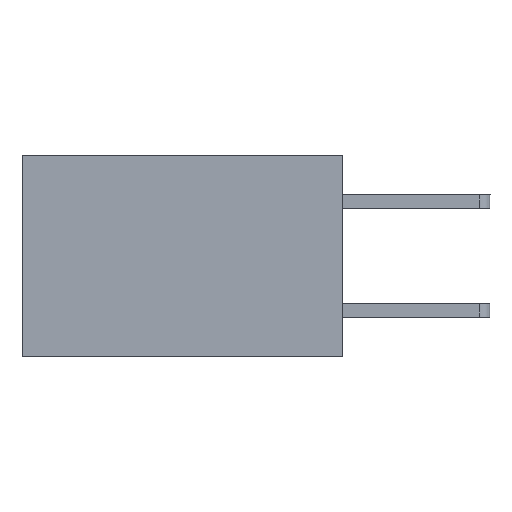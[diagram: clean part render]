
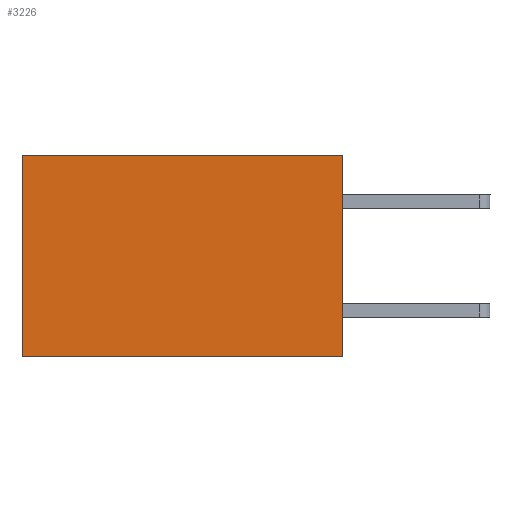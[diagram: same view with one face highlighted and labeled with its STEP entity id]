
A CAD part, left-side view. The second image highlights one B-rep face of the part: STEP entity #3226.
In plain terms, the highlighted planar face has unit normal (-1, 0, 0).
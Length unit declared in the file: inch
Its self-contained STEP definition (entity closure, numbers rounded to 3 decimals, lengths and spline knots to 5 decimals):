
#123 = VERTEX_POINT ( 'NONE', #6169 ) ;
#175 = ORIENTED_EDGE ( 'NONE', *, *, #2230, .F. ) ;
#554 = AXIS2_PLACEMENT_3D ( 'NONE', #2821, #1370, #6584 ) ;
#689 = EDGE_CURVE ( 'NONE', #6667, #6531, #8534, .T. ) ;
#781 = VECTOR ( 'NONE', #4967, 39.37008 ) ;
#1237 = ORIENTED_EDGE ( 'NONE', *, *, #689, .F. ) ;
#1370 = DIRECTION ( 'NONE',  ( 1., 0., 0. ) ) ;
#1615 = EDGE_CURVE ( 'NONE', #9536, #123, #8432, .T. ) ;
#1829 = VECTOR ( 'NONE', #3370, 39.37008 ) ;
#1859 = DIRECTION ( 'NONE',  ( 0., 1., 0. ) ) ;
#2230 = EDGE_CURVE ( 'NONE', #9536, #6667, #6528, .T. ) ;
#2776 = PLANE ( 'NONE',  #554 ) ;
#2821 = CARTESIAN_POINT ( 'NONE',  ( 0.277, 0., -0.37 ) ) ;
#3050 = EDGE_LOOP ( 'NONE', ( #4140, #1237, #175, #8078 ) ) ;
#3226 = ADVANCED_FACE ( 'NONE', ( #6485 ), #2776, .F. ) ;
#3370 = DIRECTION ( 'NONE',  ( 0., 1., 0. ) ) ;
#3591 = VECTOR ( 'NONE', #8029, 39.37008 ) ;
#4006 = CARTESIAN_POINT ( 'NONE',  ( 0.277, 0., -0.37 ) ) ;
#4068 = CARTESIAN_POINT ( 'NONE',  ( 0.277, 0.59, -0.37 ) ) ;
#4140 = ORIENTED_EDGE ( 'NONE', *, *, #8469, .T. ) ;
#4776 = CARTESIAN_POINT ( 'NONE',  ( 0.277, 0.59, -0.37 ) ) ;
#4967 = DIRECTION ( 'NONE',  ( 0., 0., -1. ) ) ;
#6169 = CARTESIAN_POINT ( 'NONE',  ( 0.277, 0.59, 0. ) ) ;
#6302 = LINE ( 'NONE', #4776, #781 ) ;
#6472 = CARTESIAN_POINT ( 'NONE',  ( 0.277, 0., -0.37 ) ) ;
#6485 = FACE_OUTER_BOUND ( 'NONE', #3050, .T. ) ;
#6528 = LINE ( 'NONE', #6472, #3591 ) ;
#6531 = VERTEX_POINT ( 'NONE', #4068 ) ;
#6561 = CARTESIAN_POINT ( 'NONE',  ( 0.277, 0., -0.37 ) ) ;
#6584 = DIRECTION ( 'NONE',  ( 0., 0., -1. ) ) ;
#6667 = VERTEX_POINT ( 'NONE', #6561 ) ;
#6758 = CARTESIAN_POINT ( 'NONE',  ( 0.277, 0., 0. ) ) ;
#8029 = DIRECTION ( 'NONE',  ( 0., 0., -1. ) ) ;
#8078 = ORIENTED_EDGE ( 'NONE', *, *, #1615, .T. ) ;
#8432 = LINE ( 'NONE', #9252, #9496 ) ;
#8469 = EDGE_CURVE ( 'NONE', #123, #6531, #6302, .T. ) ;
#8534 = LINE ( 'NONE', #4006, #1829 ) ;
#9252 = CARTESIAN_POINT ( 'NONE',  ( 0.277, 0., 0. ) ) ;
#9496 = VECTOR ( 'NONE', #1859, 39.37008 ) ;
#9536 = VERTEX_POINT ( 'NONE', #6758 ) ;
